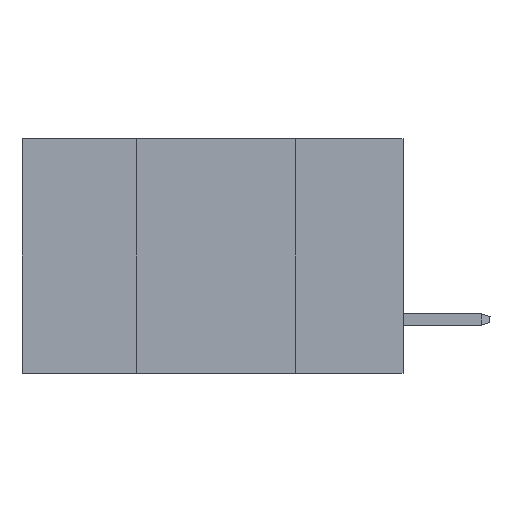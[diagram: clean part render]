
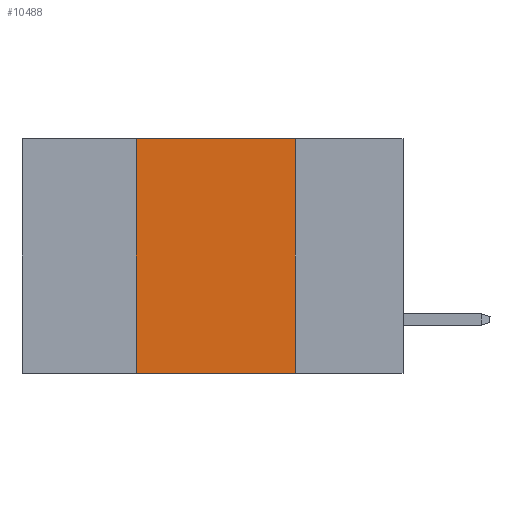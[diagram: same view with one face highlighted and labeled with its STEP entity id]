
A CAD part, left-side view. The second image highlights one B-rep face of the part: STEP entity #10488.
In plain terms, the highlighted planar face has unit normal (-1, 0, 0).
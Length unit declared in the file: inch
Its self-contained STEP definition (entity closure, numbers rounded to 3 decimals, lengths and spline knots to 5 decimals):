
#2525 = DIRECTION ( 'NONE',  ( 0., 0., -1. ) ) ;
#2536 = DIRECTION ( 'NONE',  ( 0., -1., 0. ) ) ;
#5010 = VECTOR ( 'NONE', #2536, 39.37008 ) ;
#5938 = ORIENTED_EDGE ( 'NONE', *, *, #28629, .T. ) ;
#6368 = DIRECTION ( 'NONE',  ( 0., 0., -1. ) ) ;
#6546 = LINE ( 'NONE', #15095, #13604 ) ;
#7401 = CARTESIAN_POINT ( 'NONE',  ( 0., 0.17, 0. ) ) ;
#7544 = FACE_OUTER_BOUND ( 'NONE', #9591, .T. ) ;
#8242 = ORIENTED_EDGE ( 'NONE', *, *, #34434, .F. ) ;
#9591 = EDGE_LOOP ( 'NONE', ( #16738, #8242, #16554, #5938 ) ) ;
#10255 = DIRECTION ( 'NONE',  ( 0., -1., 0. ) ) ;
#10488 = ADVANCED_FACE ( 'NONE', ( #7544 ), #18867, .F. ) ;
#13599 = DIRECTION ( 'NONE',  ( 0., 0., 1. ) ) ;
#13604 = VECTOR ( 'NONE', #6368, 39.37008 ) ;
#15095 = CARTESIAN_POINT ( 'NONE',  ( 0., 0.17, 0. ) ) ;
#15653 = VECTOR ( 'NONE', #10255, 39.37008 ) ;
#16284 = CARTESIAN_POINT ( 'NONE',  ( 0., 0.6, -0.37 ) ) ;
#16470 = LINE ( 'NONE', #16284, #5010 ) ;
#16554 = ORIENTED_EDGE ( 'NONE', *, *, #25870, .F. ) ;
#16738 = ORIENTED_EDGE ( 'NONE', *, *, #21143, .F. ) ;
#17073 = CARTESIAN_POINT ( 'NONE',  ( 0., 0.42, 0. ) ) ;
#18867 = PLANE ( 'NONE',  #30772 ) ;
#19174 = VERTEX_POINT ( 'NONE', #7401 ) ;
#19417 = DIRECTION ( 'NONE',  ( 1., 0., 0. ) ) ;
#21143 = EDGE_CURVE ( 'NONE', #19174, #28744, #6546, .T. ) ;
#22586 = CARTESIAN_POINT ( 'NONE',  ( 0., 0.17, -0.37 ) ) ;
#23926 = CARTESIAN_POINT ( 'NONE',  ( 0., 0.42, -0.37 ) ) ;
#24378 = LINE ( 'NONE', #26984, #15653 ) ;
#25870 = EDGE_CURVE ( 'NONE', #28512, #30001, #27917, .T. ) ;
#26984 = CARTESIAN_POINT ( 'NONE',  ( 0., 0.6, 0. ) ) ;
#27622 = CARTESIAN_POINT ( 'NONE',  ( 0., 0.6, 0. ) ) ;
#27917 = LINE ( 'NONE', #36297, #36366 ) ;
#28512 = VERTEX_POINT ( 'NONE', #23926 ) ;
#28629 = EDGE_CURVE ( 'NONE', #28512, #28744, #16470, .T. ) ;
#28744 = VERTEX_POINT ( 'NONE', #22586 ) ;
#30001 = VERTEX_POINT ( 'NONE', #17073 ) ;
#30772 = AXIS2_PLACEMENT_3D ( 'NONE', #27622, #19417, #2525 ) ;
#34434 = EDGE_CURVE ( 'NONE', #30001, #19174, #24378, .T. ) ;
#36297 = CARTESIAN_POINT ( 'NONE',  ( 0., 0.42, 0. ) ) ;
#36366 = VECTOR ( 'NONE', #13599, 39.37008 ) ;
